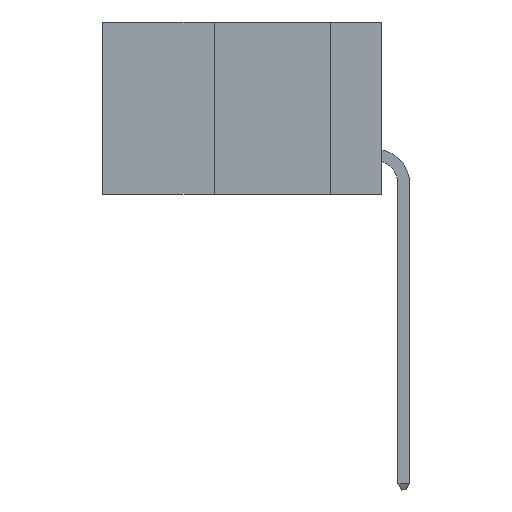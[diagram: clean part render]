
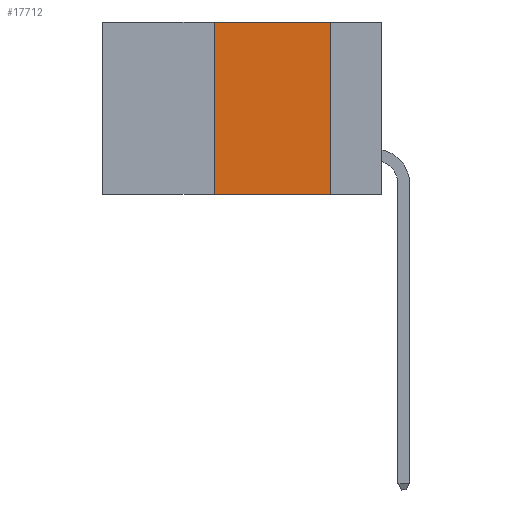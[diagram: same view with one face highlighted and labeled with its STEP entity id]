
A CAD part, left-side view. The second image highlights one B-rep face of the part: STEP entity #17712.
In plain terms, the highlighted planar face has unit normal (-1, 0, 0).
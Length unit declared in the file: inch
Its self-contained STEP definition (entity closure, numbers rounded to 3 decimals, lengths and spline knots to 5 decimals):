
#409 = CARTESIAN_POINT ( 'NONE',  ( 0., 0.36, 0. ) ) ;
#701 = EDGE_CURVE ( 'NONE', #17172, #12791, #2276, .T. ) ;
#1291 = VECTOR ( 'NONE', #17785, 39.37008 ) ;
#1564 = CARTESIAN_POINT ( 'NONE',  ( 0., 0.6, -0.37 ) ) ;
#1708 = CARTESIAN_POINT ( 'NONE',  ( 0., 0.11, -0.37 ) ) ;
#1874 = EDGE_CURVE ( 'NONE', #12791, #9809, #9706, .T. ) ;
#2276 = LINE ( 'NONE', #11641, #5484 ) ;
#2337 = ORIENTED_EDGE ( 'NONE', *, *, #5625, .T. ) ;
#2953 = AXIS2_PLACEMENT_3D ( 'NONE', #12602, #11222, #7064 ) ;
#3249 = EDGE_CURVE ( 'NONE', #9809, #5381, #8548, .T. ) ;
#3998 = ORIENTED_EDGE ( 'NONE', *, *, #701, .F. ) ;
#5381 = VERTEX_POINT ( 'NONE', #1708 ) ;
#5484 = VECTOR ( 'NONE', #14301, 39.37008 ) ;
#5625 = EDGE_CURVE ( 'NONE', #17172, #5381, #13666, .T. ) ;
#6459 = VECTOR ( 'NONE', #13165, 39.37008 ) ;
#7002 = PLANE ( 'NONE',  #2953 ) ;
#7015 = ORIENTED_EDGE ( 'NONE', *, *, #3249, .F. ) ;
#7064 = DIRECTION ( 'NONE',  ( 0., 0., -1. ) ) ;
#7649 = CARTESIAN_POINT ( 'NONE',  ( 0., 0.6, 0. ) ) ;
#8548 = LINE ( 'NONE', #11988, #18085 ) ;
#9706 = LINE ( 'NONE', #7649, #1291 ) ;
#9809 = VERTEX_POINT ( 'NONE', #11710 ) ;
#11222 = DIRECTION ( 'NONE',  ( 1., 0., 0. ) ) ;
#11641 = CARTESIAN_POINT ( 'NONE',  ( 0., 0.36, 0. ) ) ;
#11710 = CARTESIAN_POINT ( 'NONE',  ( 0., 0.11, 0. ) ) ;
#11988 = CARTESIAN_POINT ( 'NONE',  ( 0., 0.11, 0. ) ) ;
#12602 = CARTESIAN_POINT ( 'NONE',  ( 0., 0.6, 0. ) ) ;
#12791 = VERTEX_POINT ( 'NONE', #409 ) ;
#13165 = DIRECTION ( 'NONE',  ( 0., -1., 0. ) ) ;
#13380 = EDGE_LOOP ( 'NONE', ( #7015, #17753, #3998, #2337 ) ) ;
#13666 = LINE ( 'NONE', #1564, #6459 ) ;
#14301 = DIRECTION ( 'NONE',  ( 0., 0., 1. ) ) ;
#15025 = DIRECTION ( 'NONE',  ( 0., 0., -1. ) ) ;
#16512 = FACE_OUTER_BOUND ( 'NONE', #13380, .T. ) ;
#17172 = VERTEX_POINT ( 'NONE', #17284 ) ;
#17284 = CARTESIAN_POINT ( 'NONE',  ( 0., 0.36, -0.37 ) ) ;
#17712 = ADVANCED_FACE ( 'NONE', ( #16512 ), #7002, .F. ) ;
#17753 = ORIENTED_EDGE ( 'NONE', *, *, #1874, .F. ) ;
#17785 = DIRECTION ( 'NONE',  ( 0., -1., 0. ) ) ;
#18085 = VECTOR ( 'NONE', #15025, 39.37008 ) ;
